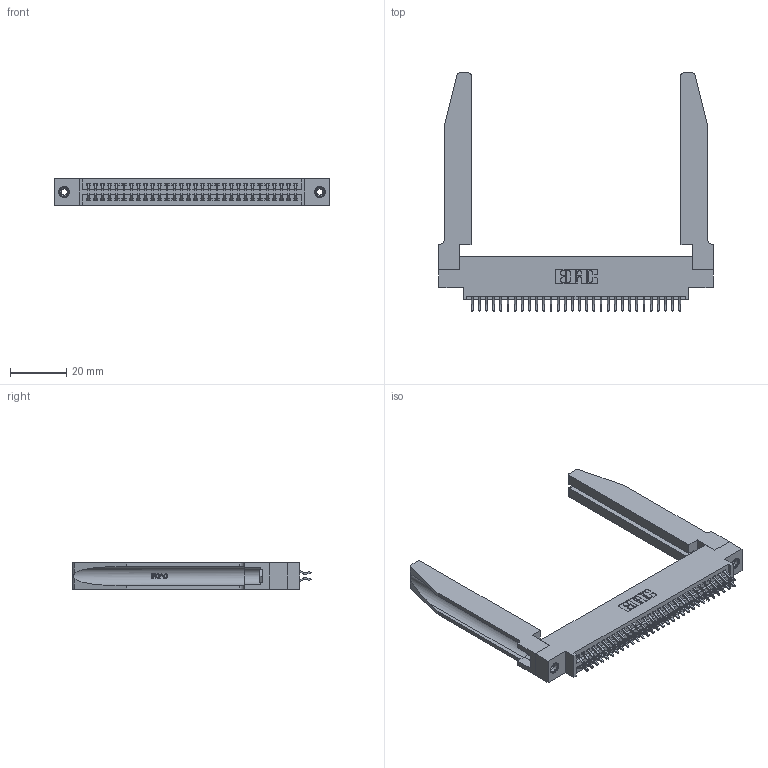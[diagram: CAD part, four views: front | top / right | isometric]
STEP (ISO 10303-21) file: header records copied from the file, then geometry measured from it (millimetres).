
FILE_DESCRIPTION (( 'STEP AP203' ), '1' );
FILE_NAME ('395-060-556-878.STEP', '2019-10-23T14:50:27', ( '' ), ( '' ), 'SwSTEP 2.0', 'SolidWorks 2016', '' );
FILE_SCHEMA (( 'CONFIG_CONTROL_DESIGN' ));
Length unit declared in the file: inch
Products named in the file (5): 395-060-556-878; 345 Part_0.170 Offset - 0.156 Dia-TH; 345-292-001_556 Tail; 345-250-001_345-250-001-102; 345-220-078_345-220-078
Assembly tree (65 placements, depth 2):
  395-060-556-878
    345 Part_0.170 Offset - 0.156 Dia-TH
    345-292-001_556 Tail  x60
    345-250-001_345-250-001-102  x2
    345-220-078_345-220-078  x2
Bounding box: 97.43 x 84.51 x 9.4 mm (x, y, z)
Volume: 17008.2 mm3; surface area: 20351.9 mm2
Topology: 65 solids, 65 shells, 3724 faces, 10981 edges, 7230 vertices
Faces by surface type: plane 2446, cylinder 1226, bspline 36, cone 12, torus 4
Entity records: 30246 total; most frequent: CARTESIAN_POINT 6015, ORIENTED_EDGE 4834, DIRECTION 4299, EDGE_CURVE 2417, VECTOR 2063, LINE 2063, VERTEX_POINT 1604, AXIS2_PLACEMENT_3D 1118
